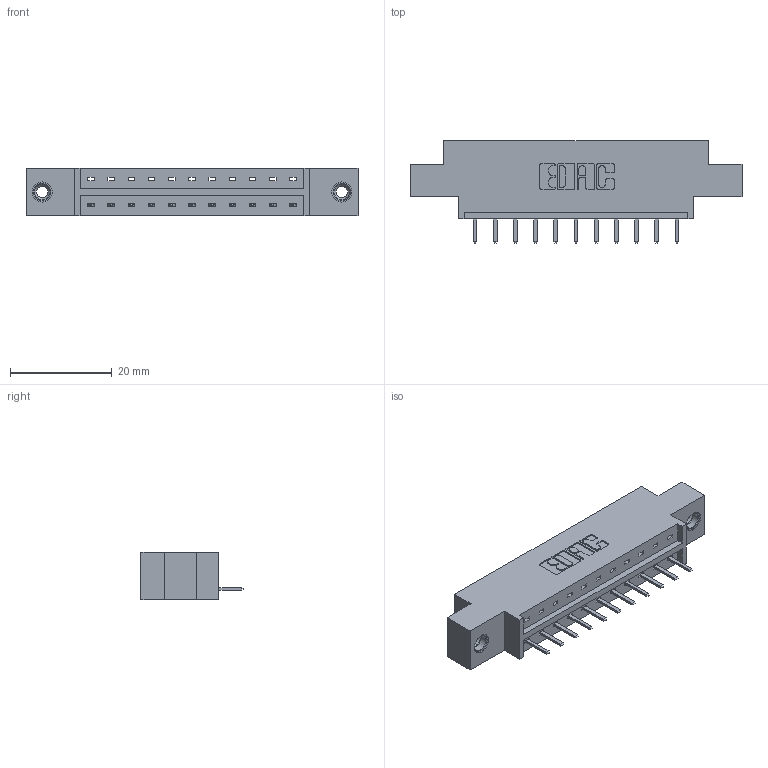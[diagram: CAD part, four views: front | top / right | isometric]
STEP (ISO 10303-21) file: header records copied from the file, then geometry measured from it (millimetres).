
FILE_DESCRIPTION (( 'STEP AP203' ), '1' );
FILE_NAME ('333-011-520-608.STEP', '2018-07-31T23:18:47', ( '' ), ( '' ), 'SwSTEP 2.0', 'SolidWorks 2016', '' );
FILE_SCHEMA (( 'CONFIG_CONTROL_DESIGN' ));
Length unit declared in the file: inch
Products named in the file (4): 333 Part_Offset - .156 Dia - TI; 345-292-001_345-293-120; 345-250-001_345-250-003-102; 333-011-520-608
Assembly tree (14 placements, depth 2):
  333-011-520-608
    333 Part_Offset - .156 Dia - TI
    345-292-001_345-293-120  x11
    345-250-001_345-250-003-102  x2
Bounding box: 65.13 x 20.02 x 9.4 mm (x, y, z)
Volume: 6020.9 mm3; surface area: 6424.4 mm2
Topology: 14 solids, 14 shells, 860 faces, 2483 edges, 1618 vertices
Faces by surface type: plane 590, cylinder 254, cone 12, torus 4
Entity records: 12166 total; most frequent: CARTESIAN_POINT 2098, ORIENTED_EDGE 2026, DIRECTION 1853, EDGE_CURVE 1013, VECTOR 861, LINE 861, VERTEX_POINT 668, AXIS2_PLACEMENT_3D 496
